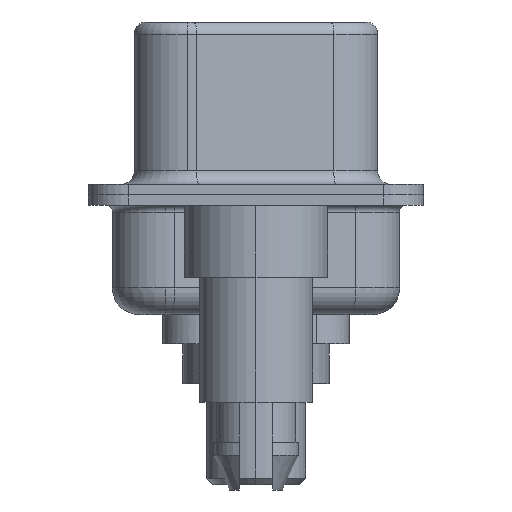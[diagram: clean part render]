
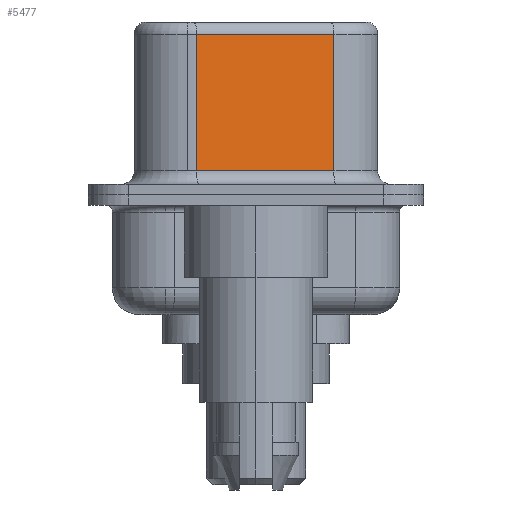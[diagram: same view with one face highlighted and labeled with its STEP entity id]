
A CAD part, left-side view. The second image highlights one B-rep face of the part: STEP entity #5477.
In plain terms, the highlighted planar face has unit normal (-0.985, -0.174, 0).
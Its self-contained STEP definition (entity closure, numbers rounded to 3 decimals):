
#475 = LINE ( 'NONE', #12144, #2802 ) ;
#1562 = DIRECTION ( 'NONE',  ( 0., 0., -1. ) ) ;
#1867 = VECTOR ( 'NONE', #4837, 1000. ) ;
#2347 = DIRECTION ( 'NONE',  ( 0., 0., -1. ) ) ;
#2802 = VECTOR ( 'NONE', #3796, 1000. ) ;
#2810 = LINE ( 'NONE', #8414, #14697 ) ;
#3367 = VERTEX_POINT ( 'NONE', #6875 ) ;
#3662 = EDGE_CURVE ( 'NONE', #4224, #3367, #2810, .T. ) ;
#3796 = DIRECTION ( 'NONE',  ( 0.174, -0.985, 0. ) ) ;
#3976 = VECTOR ( 'NONE', #2347, 1000. ) ;
#4224 = VERTEX_POINT ( 'NONE', #13681 ) ;
#4837 = DIRECTION ( 'NONE',  ( -0.174, 0.985, 0. ) ) ;
#5117 = ORIENTED_EDGE ( 'NONE', *, *, #6785, .F. ) ;
#5477 = ADVANCED_FACE ( 'NONE', ( #10809 ), #10881, .F. ) ;
#6113 = CARTESIAN_POINT ( 'NONE',  ( 4.585, -2.927, 6.02 ) ) ;
#6785 = EDGE_CURVE ( 'NONE', #10876, #13774, #13507, .T. ) ;
#6875 = CARTESIAN_POINT ( 'NONE',  ( 3.675, 2.233, 0.9 ) ) ;
#7072 = EDGE_LOOP ( 'NONE', ( #5117, #12085, #14612, #9507 ) ) ;
#8414 = CARTESIAN_POINT ( 'NONE',  ( 3.675, 2.233, 6.52 ) ) ;
#9507 = ORIENTED_EDGE ( 'NONE', *, *, #10263, .T. ) ;
#9621 = CARTESIAN_POINT ( 'NONE',  ( 4.585, -2.927, 6.02 ) ) ;
#10263 = EDGE_CURVE ( 'NONE', #3367, #13774, #475, .T. ) ;
#10809 = FACE_OUTER_BOUND ( 'NONE', #7072, .T. ) ;
#10871 = CARTESIAN_POINT ( 'NONE',  ( 4.585, -2.927, 0.9 ) ) ;
#10876 = VERTEX_POINT ( 'NONE', #6113 ) ;
#10881 = PLANE ( 'NONE',  #15172 ) ;
#10898 = DIRECTION ( 'NONE',  ( 0.985, 0.174, 0. ) ) ;
#11316 = LINE ( 'NONE', #9621, #1867 ) ;
#12085 = ORIENTED_EDGE ( 'NONE', *, *, #13091, .T. ) ;
#12111 = DIRECTION ( 'NONE',  ( -0.174, 0.985, 0. ) ) ;
#12144 = CARTESIAN_POINT ( 'NONE',  ( 4.585, -2.927, 0.9 ) ) ;
#12811 = CARTESIAN_POINT ( 'NONE',  ( 4.585, -2.927, 6.52 ) ) ;
#13091 = EDGE_CURVE ( 'NONE', #10876, #4224, #11316, .T. ) ;
#13507 = LINE ( 'NONE', #12811, #3976 ) ;
#13681 = CARTESIAN_POINT ( 'NONE',  ( 3.675, 2.233, 6.02 ) ) ;
#13774 = VERTEX_POINT ( 'NONE', #10871 ) ;
#13954 = CARTESIAN_POINT ( 'NONE',  ( 4.585, -2.927, 6.52 ) ) ;
#14612 = ORIENTED_EDGE ( 'NONE', *, *, #3662, .T. ) ;
#14697 = VECTOR ( 'NONE', #1562, 1000. ) ;
#15172 = AXIS2_PLACEMENT_3D ( 'NONE', #13954, #10898, #12111 ) ;
